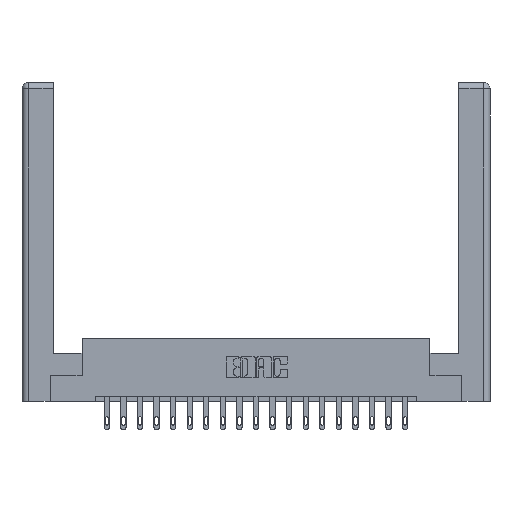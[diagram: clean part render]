
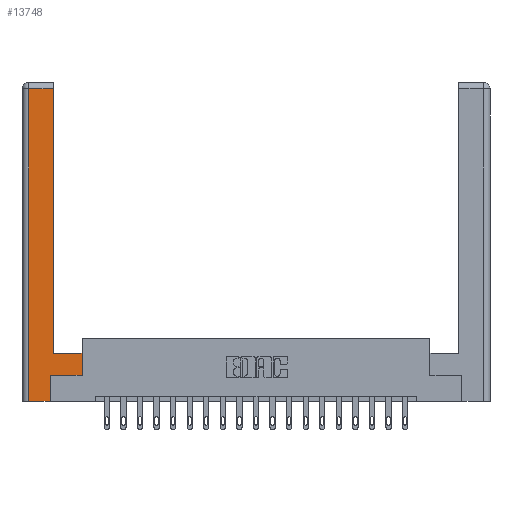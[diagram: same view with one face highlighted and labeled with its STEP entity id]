
A CAD part, top view. The second image highlights one B-rep face of the part: STEP entity #13748.
In plain terms, the highlighted planar face has unit normal (0, 0, 1).
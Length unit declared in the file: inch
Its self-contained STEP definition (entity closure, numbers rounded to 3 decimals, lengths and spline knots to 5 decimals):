
#362 = ORIENTED_EDGE ( 'NONE', *, *, #2986, .T. ) ;
#702 = CARTESIAN_POINT ( 'NONE',  ( 0.0615, 2.94, 0. ) ) ;
#717 = EDGE_CURVE ( 'NONE', #1087, #19518, #9439, .T. ) ;
#1087 = VERTEX_POINT ( 'NONE', #2927 ) ;
#1208 = ORIENTED_EDGE ( 'NONE', *, *, #6294, .T. ) ;
#1693 = VERTEX_POINT ( 'NONE', #4477 ) ;
#1816 = ORIENTED_EDGE ( 'NONE', *, *, #18821, .T. ) ;
#1922 = PLANE ( 'NONE',  #18367 ) ;
#2037 = CARTESIAN_POINT ( 'NONE',  ( 0.265, 0., 0. ) ) ;
#2054 = CARTESIAN_POINT ( 'NONE',  ( 0., 0., 0. ) ) ;
#2646 = CARTESIAN_POINT ( 'NONE',  ( 0.0615, 2.94, 0. ) ) ;
#2711 = LINE ( 'NONE', #15311, #4919 ) ;
#2899 = CARTESIAN_POINT ( 'NONE',  ( 0.295, 2.94, 0. ) ) ;
#2927 = CARTESIAN_POINT ( 'NONE',  ( 0.295, 0.45, 0. ) ) ;
#2986 = EDGE_CURVE ( 'NONE', #14252, #12595, #11076, .T. ) ;
#3377 = LINE ( 'NONE', #18336, #8514 ) ;
#3387 = EDGE_CURVE ( 'NONE', #12595, #18955, #10013, .T. ) ;
#3552 = LINE ( 'NONE', #8351, #4791 ) ;
#4306 = DIRECTION ( 'NONE',  ( 1., 0., 0. ) ) ;
#4353 = VECTOR ( 'NONE', #8264, 39.37008 ) ;
#4477 = CARTESIAN_POINT ( 'NONE',  ( 0.565, 0.45, 0. ) ) ;
#4791 = VECTOR ( 'NONE', #10022, 39.37008 ) ;
#4919 = VECTOR ( 'NONE', #6491, 39.37008 ) ;
#5396 = LINE ( 'NONE', #9659, #6863 ) ;
#6294 = EDGE_CURVE ( 'NONE', #19518, #16961, #12585, .T. ) ;
#6491 = DIRECTION ( 'NONE',  ( 0., 1., 0. ) ) ;
#6863 = VECTOR ( 'NONE', #14319, 39.37008 ) ;
#7832 = EDGE_LOOP ( 'NONE', ( #14582, #1208, #19458, #10985, #362, #16238, #1816, #19308 ) ) ;
#8080 = DIRECTION ( 'NONE',  ( 0., 0., -1. ) ) ;
#8264 = DIRECTION ( 'NONE',  ( 1., 0., 0. ) ) ;
#8336 = DIRECTION ( 'NONE',  ( 0., 1., 0. ) ) ;
#8351 = CARTESIAN_POINT ( 'NONE',  ( 0.295, 0.45, 0. ) ) ;
#8514 = VECTOR ( 'NONE', #4306, 39.37008 ) ;
#8585 = DIRECTION ( 'NONE',  ( -1., 0., 0. ) ) ;
#8913 = VECTOR ( 'NONE', #8585, 39.37008 ) ;
#9366 = CARTESIAN_POINT ( 'NONE',  ( 0.265, 0.245, 0. ) ) ;
#9439 = LINE ( 'NONE', #14791, #16787 ) ;
#9659 = CARTESIAN_POINT ( 'NONE',  ( 0.0615, 0., 0. ) ) ;
#10013 = LINE ( 'NONE', #11371, #4353 ) ;
#10022 = DIRECTION ( 'NONE',  ( -1., 0., 0. ) ) ;
#10985 = ORIENTED_EDGE ( 'NONE', *, *, #20068, .T. ) ;
#11048 = VERTEX_POINT ( 'NONE', #11999 ) ;
#11076 = LINE ( 'NONE', #9366, #17905 ) ;
#11371 = CARTESIAN_POINT ( 'NONE',  ( 0.565, 0.245, 0. ) ) ;
#11473 = EDGE_CURVE ( 'NONE', #16961, #11048, #5396, .T. ) ;
#11999 = CARTESIAN_POINT ( 'NONE',  ( 0.0615, 0., 0. ) ) ;
#12585 = LINE ( 'NONE', #702, #8913 ) ;
#12595 = VERTEX_POINT ( 'NONE', #19874 ) ;
#13748 = ADVANCED_FACE ( 'NONE', ( #16075 ), #1922, .F. ) ;
#13972 = DIRECTION ( 'NONE',  ( 0., 1., 0. ) ) ;
#14252 = VERTEX_POINT ( 'NONE', #2037 ) ;
#14319 = DIRECTION ( 'NONE',  ( 0., -1., 0. ) ) ;
#14582 = ORIENTED_EDGE ( 'NONE', *, *, #717, .T. ) ;
#14791 = CARTESIAN_POINT ( 'NONE',  ( 0.295, 3., 0. ) ) ;
#15311 = CARTESIAN_POINT ( 'NONE',  ( 0.565, 0.45, 0. ) ) ;
#16075 = FACE_OUTER_BOUND ( 'NONE', #7832, .T. ) ;
#16116 = EDGE_CURVE ( 'NONE', #1693, #1087, #3552, .T. ) ;
#16238 = ORIENTED_EDGE ( 'NONE', *, *, #3387, .T. ) ;
#16787 = VECTOR ( 'NONE', #8336, 39.37008 ) ;
#16961 = VERTEX_POINT ( 'NONE', #2646 ) ;
#17905 = VECTOR ( 'NONE', #13972, 39.37008 ) ;
#18336 = CARTESIAN_POINT ( 'NONE',  ( 0.265, 0., 0. ) ) ;
#18367 = AXIS2_PLACEMENT_3D ( 'NONE', #2054, #8080, #19025 ) ;
#18821 = EDGE_CURVE ( 'NONE', #18955, #1693, #2711, .T. ) ;
#18955 = VERTEX_POINT ( 'NONE', #19188 ) ;
#19025 = DIRECTION ( 'NONE',  ( -1., 0., 0. ) ) ;
#19188 = CARTESIAN_POINT ( 'NONE',  ( 0.565, 0.245, 0. ) ) ;
#19308 = ORIENTED_EDGE ( 'NONE', *, *, #16116, .T. ) ;
#19458 = ORIENTED_EDGE ( 'NONE', *, *, #11473, .T. ) ;
#19518 = VERTEX_POINT ( 'NONE', #2899 ) ;
#19874 = CARTESIAN_POINT ( 'NONE',  ( 0.265, 0.245, 0. ) ) ;
#20068 = EDGE_CURVE ( 'NONE', #11048, #14252, #3377, .T. ) ;
